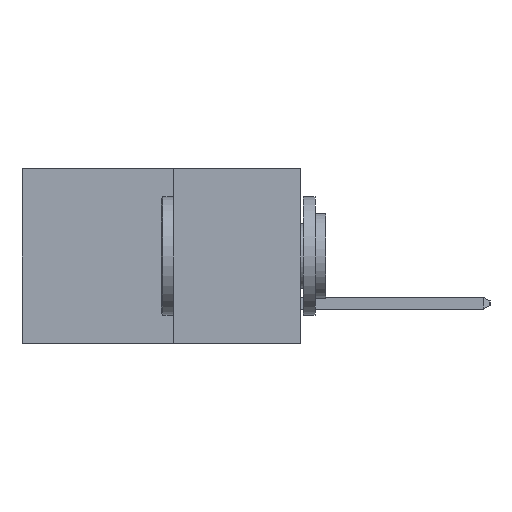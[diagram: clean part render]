
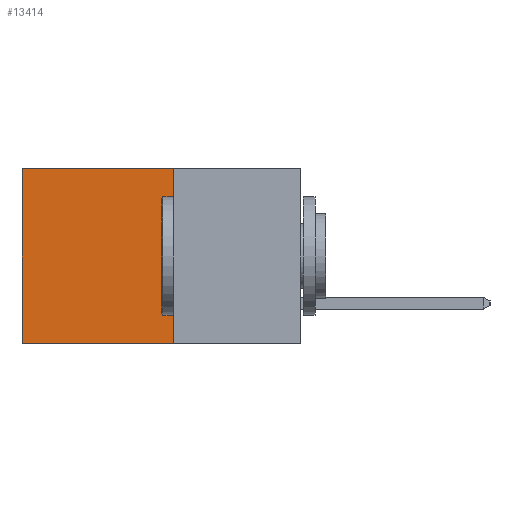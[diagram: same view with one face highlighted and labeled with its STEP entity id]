
A CAD part, left-side view. The second image highlights one B-rep face of the part: STEP entity #13414.
In plain terms, the highlighted planar face has unit normal (-1, 0, 0).
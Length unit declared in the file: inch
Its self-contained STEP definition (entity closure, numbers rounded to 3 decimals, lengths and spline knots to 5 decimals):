
#118 = AXIS2_PLACEMENT_3D ( 'NONE', #13861, #8073, #21692 ) ;
#1029 = EDGE_CURVE ( 'NONE', #10242, #7106, #18681, .T. ) ;
#1864 = EDGE_CURVE ( 'NONE', #5434, #3315, #22824, .T. ) ;
#2052 = VECTOR ( 'NONE', #24332, 39.37008 ) ;
#2245 = LINE ( 'NONE', #19375, #22416 ) ;
#2345 = CARTESIAN_POINT ( 'NONE',  ( 0.277, 0.59, 0. ) ) ;
#2678 = ORIENTED_EDGE ( 'NONE', *, *, #1864, .F. ) ;
#3315 = VERTEX_POINT ( 'NONE', #17817 ) ;
#3714 = CARTESIAN_POINT ( 'NONE',  ( 0.277, 0.27, -0.37 ) ) ;
#3764 = EDGE_CURVE ( 'NONE', #7106, #3315, #2245, .T. ) ;
#5434 = VERTEX_POINT ( 'NONE', #8176 ) ;
#6239 = DIRECTION ( 'NONE',  ( 0., 0., -1. ) ) ;
#7106 = VERTEX_POINT ( 'NONE', #2345 ) ;
#8073 = DIRECTION ( 'NONE',  ( 1., 0., 0. ) ) ;
#8176 = CARTESIAN_POINT ( 'NONE',  ( 0.277, 0.27, -0.37 ) ) ;
#8501 = EDGE_CURVE ( 'NONE', #10242, #5434, #21159, .T. ) ;
#10242 = VERTEX_POINT ( 'NONE', #15231 ) ;
#10541 = DIRECTION ( 'NONE',  ( 0., 1., 0. ) ) ;
#12431 = CARTESIAN_POINT ( 'NONE',  ( 0.277, 0.27, 0. ) ) ;
#13414 = ADVANCED_FACE ( 'NONE', ( #25206 ), #19752, .F. ) ;
#13861 = CARTESIAN_POINT ( 'NONE',  ( 0.277, 0.27, -0.37 ) ) ;
#14125 = VECTOR ( 'NONE', #6239, 39.37008 ) ;
#15231 = CARTESIAN_POINT ( 'NONE',  ( 0.277, 0.27, 0. ) ) ;
#15997 = CARTESIAN_POINT ( 'NONE',  ( 0.277, 0.27, -0.37 ) ) ;
#17817 = CARTESIAN_POINT ( 'NONE',  ( 0.277, 0.59, -0.37 ) ) ;
#18057 = VECTOR ( 'NONE', #10541, 39.37008 ) ;
#18534 = DIRECTION ( 'NONE',  ( 0., 0., -1. ) ) ;
#18681 = LINE ( 'NONE', #12431, #18057 ) ;
#19375 = CARTESIAN_POINT ( 'NONE',  ( 0.277, 0.59, -0.37 ) ) ;
#19752 = PLANE ( 'NONE',  #118 ) ;
#19792 = ORIENTED_EDGE ( 'NONE', *, *, #1029, .T. ) ;
#21159 = LINE ( 'NONE', #15997, #14125 ) ;
#21692 = DIRECTION ( 'NONE',  ( 0., 0., -1. ) ) ;
#22416 = VECTOR ( 'NONE', #18534, 39.37008 ) ;
#22452 = ORIENTED_EDGE ( 'NONE', *, *, #3764, .T. ) ;
#22549 = ORIENTED_EDGE ( 'NONE', *, *, #8501, .F. ) ;
#22824 = LINE ( 'NONE', #3714, #2052 ) ;
#22932 = EDGE_LOOP ( 'NONE', ( #22452, #2678, #22549, #19792 ) ) ;
#24332 = DIRECTION ( 'NONE',  ( 0., 1., 0. ) ) ;
#25206 = FACE_OUTER_BOUND ( 'NONE', #22932, .T. ) ;
